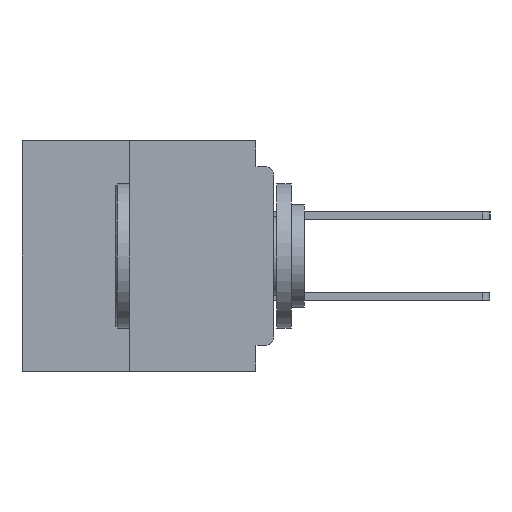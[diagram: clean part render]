
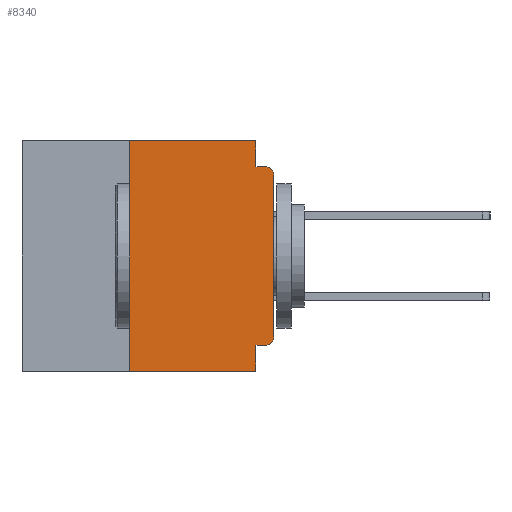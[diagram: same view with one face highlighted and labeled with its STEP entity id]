
A CAD part, left-side view. The second image highlights one B-rep face of the part: STEP entity #8340.
In plain terms, the highlighted planar face has unit normal (-1, 0, 0).
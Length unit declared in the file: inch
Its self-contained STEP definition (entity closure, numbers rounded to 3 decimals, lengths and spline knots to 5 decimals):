
#394 = LINE ( 'NONE', #30248, #36403 ) ;
#944 = VERTEX_POINT ( 'NONE', #6037 ) ;
#1087 = ORIENTED_EDGE ( 'NONE', *, *, #35653, .F. ) ;
#1535 = DIRECTION ( 'NONE',  ( 0., 0., -1. ) ) ;
#2139 = VERTEX_POINT ( 'NONE', #27295 ) ;
#2547 = CARTESIAN_POINT ( 'NONE',  ( 0., 0.25, -0.4 ) ) ;
#3222 = EDGE_CURVE ( 'NONE', #2139, #12713, #28824, .T. ) ;
#3412 = ORIENTED_EDGE ( 'NONE', *, *, #16378, .F. ) ;
#3602 = VERTEX_POINT ( 'NONE', #29616 ) ;
#4061 = LINE ( 'NONE', #34833, #33427 ) ;
#6037 = CARTESIAN_POINT ( 'NONE',  ( 0., 0.015, -0.045 ) ) ;
#6592 = ORIENTED_EDGE ( 'NONE', *, *, #3222, .F. ) ;
#6685 = AXIS2_PLACEMENT_3D ( 'NONE', #35558, #18889, #1535 ) ;
#6824 = ORIENTED_EDGE ( 'NONE', *, *, #35138, .F. ) ;
#7117 = ORIENTED_EDGE ( 'NONE', *, *, #15751, .T. ) ;
#7378 = VECTOR ( 'NONE', #20461, 39.37008 ) ;
#7419 = VECTOR ( 'NONE', #21436, 39.37008 ) ;
#8340 = ADVANCED_FACE ( 'NONE', ( #36032 ), #27598, .F. ) ;
#9855 = ORIENTED_EDGE ( 'NONE', *, *, #24050, .F. ) ;
#9972 = VECTOR ( 'NONE', #36359, 39.37008 ) ;
#10442 = DIRECTION ( 'NONE',  ( 0., -1., 0. ) ) ;
#10495 = EDGE_CURVE ( 'NONE', #14078, #27121, #32612, .T. ) ;
#11367 = DIRECTION ( 'NONE',  ( -1., 0., 0. ) ) ;
#11381 = CARTESIAN_POINT ( 'NONE',  ( 0., 0.437, 0. ) ) ;
#11704 = EDGE_CURVE ( 'NONE', #34730, #944, #13467, .T. ) ;
#11737 = CARTESIAN_POINT ( 'NONE',  ( 0., 0., -0.34 ) ) ;
#11886 = DIRECTION ( 'NONE',  ( 0., 0., -1. ) ) ;
#11924 = ORIENTED_EDGE ( 'NONE', *, *, #13465, .F. ) ;
#12324 = CARTESIAN_POINT ( 'NONE',  ( 0., 0.031, 0. ) ) ;
#12713 = VERTEX_POINT ( 'NONE', #30352 ) ;
#13465 = EDGE_CURVE ( 'NONE', #14828, #2139, #13945, .T. ) ;
#13467 = CIRCLE ( 'NONE', #30063, 0.015 ) ;
#13945 = LINE ( 'NONE', #11381, #28263 ) ;
#14078 = VERTEX_POINT ( 'NONE', #2547 ) ;
#14246 = AXIS2_PLACEMENT_3D ( 'NONE', #27358, #26869, #26837 ) ;
#14828 = VERTEX_POINT ( 'NONE', #34451 ) ;
#15751 = EDGE_CURVE ( 'NONE', #36781, #17360, #20518, .T. ) ;
#15790 = LINE ( 'NONE', #32025, #23371 ) ;
#16378 = EDGE_CURVE ( 'NONE', #3602, #27121, #23603, .T. ) ;
#17360 = VERTEX_POINT ( 'NONE', #11737 ) ;
#17612 = CARTESIAN_POINT ( 'NONE',  ( 0., 0., 0. ) ) ;
#17752 = CARTESIAN_POINT ( 'NONE',  ( 0., 0.015, -0.355 ) ) ;
#18106 = DIRECTION ( 'NONE',  ( 0., 1., 0. ) ) ;
#18889 = DIRECTION ( 'NONE',  ( -1., 0., 0. ) ) ;
#20434 = CARTESIAN_POINT ( 'NONE',  ( 0., 0., -0.06 ) ) ;
#20461 = DIRECTION ( 'NONE',  ( 0., 0., 1. ) ) ;
#20518 = CIRCLE ( 'NONE', #6685, 0.015 ) ;
#21230 = VECTOR ( 'NONE', #11886, 39.37008 ) ;
#21352 = ORIENTED_EDGE ( 'NONE', *, *, #23129, .T. ) ;
#21436 = DIRECTION ( 'NONE',  ( 0., 0., -1. ) ) ;
#22611 = CARTESIAN_POINT ( 'NONE',  ( 0., 0.437, -0.4 ) ) ;
#23129 = EDGE_CURVE ( 'NONE', #17360, #34730, #31030, .T. ) ;
#23371 = VECTOR ( 'NONE', #23428, 39.37008 ) ;
#23428 = DIRECTION ( 'NONE',  ( 0., 0., 1. ) ) ;
#23603 = LINE ( 'NONE', #32615, #7419 ) ;
#24050 = EDGE_CURVE ( 'NONE', #12713, #944, #394, .T. ) ;
#25664 = DIRECTION ( 'NONE',  ( 0., -1., 0. ) ) ;
#26837 = DIRECTION ( 'NONE',  ( 0., 0., -1. ) ) ;
#26869 = DIRECTION ( 'NONE',  ( 1., 0., 0. ) ) ;
#27121 = VERTEX_POINT ( 'NONE', #33397 ) ;
#27295 = CARTESIAN_POINT ( 'NONE',  ( 0., 0.031, 0. ) ) ;
#27358 = CARTESIAN_POINT ( 'NONE',  ( 0., 0.437, 0. ) ) ;
#27598 = PLANE ( 'NONE',  #14246 ) ;
#28263 = VECTOR ( 'NONE', #25664, 39.37008 ) ;
#28502 = CARTESIAN_POINT ( 'NONE',  ( 0., 0.015, -0.06 ) ) ;
#28613 = ORIENTED_EDGE ( 'NONE', *, *, #11704, .T. ) ;
#28706 = EDGE_LOOP ( 'NONE', ( #21352, #28613, #9855, #6592, #11924, #1087, #35118, #3412, #6824, #7117 ) ) ;
#28824 = LINE ( 'NONE', #12324, #21230 ) ;
#29616 = CARTESIAN_POINT ( 'NONE',  ( 0., 0.031, -0.355 ) ) ;
#30063 = AXIS2_PLACEMENT_3D ( 'NONE', #28502, #11367, #31274 ) ;
#30248 = CARTESIAN_POINT ( 'NONE',  ( 0., 0., -0.045 ) ) ;
#30352 = CARTESIAN_POINT ( 'NONE',  ( 0., 0.031, -0.045 ) ) ;
#31030 = LINE ( 'NONE', #17612, #7378 ) ;
#31274 = DIRECTION ( 'NONE',  ( 0., 0., -1. ) ) ;
#32025 = CARTESIAN_POINT ( 'NONE',  ( 0., 0.25, -0.4 ) ) ;
#32612 = LINE ( 'NONE', #22611, #9972 ) ;
#32615 = CARTESIAN_POINT ( 'NONE',  ( 0., 0.031, -0.4 ) ) ;
#33397 = CARTESIAN_POINT ( 'NONE',  ( 0., 0.031, -0.4 ) ) ;
#33427 = VECTOR ( 'NONE', #18106, 39.37008 ) ;
#34451 = CARTESIAN_POINT ( 'NONE',  ( 0., 0.25, 0. ) ) ;
#34730 = VERTEX_POINT ( 'NONE', #20434 ) ;
#34833 = CARTESIAN_POINT ( 'NONE',  ( 0., 0., -0.355 ) ) ;
#35118 = ORIENTED_EDGE ( 'NONE', *, *, #10495, .T. ) ;
#35138 = EDGE_CURVE ( 'NONE', #36781, #3602, #4061, .T. ) ;
#35558 = CARTESIAN_POINT ( 'NONE',  ( 0., 0.015, -0.34 ) ) ;
#35653 = EDGE_CURVE ( 'NONE', #14078, #14828, #15790, .T. ) ;
#36032 = FACE_OUTER_BOUND ( 'NONE', #28706, .T. ) ;
#36359 = DIRECTION ( 'NONE',  ( 0., -1., 0. ) ) ;
#36403 = VECTOR ( 'NONE', #10442, 39.37008 ) ;
#36781 = VERTEX_POINT ( 'NONE', #17752 ) ;
